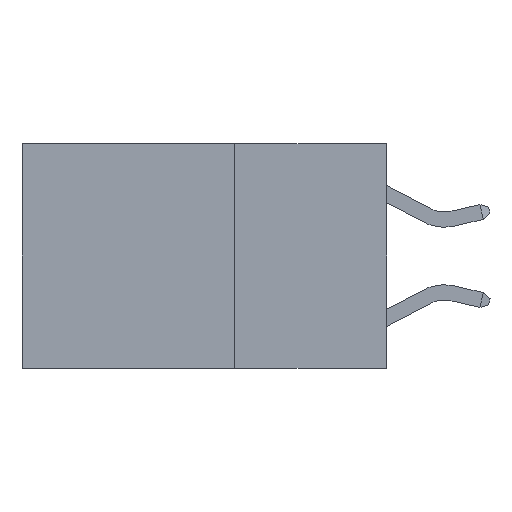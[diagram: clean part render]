
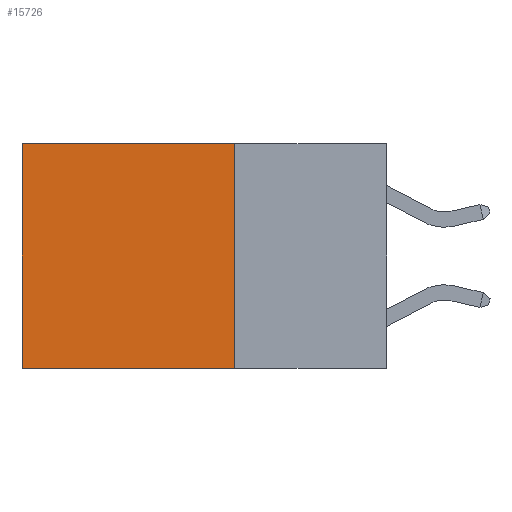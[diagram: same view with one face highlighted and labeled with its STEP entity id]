
A CAD part, left-side view. The second image highlights one B-rep face of the part: STEP entity #15726.
In plain terms, the highlighted planar face has unit normal (-1, 0, 0).
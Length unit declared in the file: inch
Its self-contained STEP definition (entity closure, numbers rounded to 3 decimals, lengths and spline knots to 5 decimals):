
#18 = DIRECTION ( 'NONE',  ( 0., 1., 0. ) ) ;
#278 = AXIS2_PLACEMENT_3D ( 'NONE', #5796, #12314, #14720 ) ;
#435 = CARTESIAN_POINT ( 'NONE',  ( 0.2625, 0.25, -0.37 ) ) ;
#825 = CARTESIAN_POINT ( 'NONE',  ( 0.2625, 0.6, 0. ) ) ;
#2890 = EDGE_CURVE ( 'NONE', #19317, #10851, #18489, .T. ) ;
#3599 = EDGE_LOOP ( 'NONE', ( #5713, #4068, #4902, #7153 ) ) ;
#4068 = ORIENTED_EDGE ( 'NONE', *, *, #8399, .F. ) ;
#4902 = ORIENTED_EDGE ( 'NONE', *, *, #13349, .F. ) ;
#5343 = VECTOR ( 'NONE', #9187, 39.37008 ) ;
#5713 = ORIENTED_EDGE ( 'NONE', *, *, #14063, .T. ) ;
#5796 = CARTESIAN_POINT ( 'NONE',  ( 0.2625, 0.25, 0. ) ) ;
#6402 = CARTESIAN_POINT ( 'NONE',  ( 0.2625, 0.25, 0. ) ) ;
#7153 = ORIENTED_EDGE ( 'NONE', *, *, #2890, .T. ) ;
#7994 = VERTEX_POINT ( 'NONE', #11801 ) ;
#8399 = EDGE_CURVE ( 'NONE', #13211, #7994, #14859, .T. ) ;
#9078 = LINE ( 'NONE', #825, #5343 ) ;
#9187 = DIRECTION ( 'NONE',  ( 0., 0., -1. ) ) ;
#10851 = VERTEX_POINT ( 'NONE', #14074 ) ;
#11346 = CARTESIAN_POINT ( 'NONE',  ( 0.2625, 0.25, 0. ) ) ;
#11454 = LINE ( 'NONE', #11346, #20994 ) ;
#11801 = CARTESIAN_POINT ( 'NONE',  ( 0.2625, 0.6, -0.37 ) ) ;
#12314 = DIRECTION ( 'NONE',  ( 1., 0., 0. ) ) ;
#13165 = DIRECTION ( 'NONE',  ( 0., 0., -1. ) ) ;
#13211 = VERTEX_POINT ( 'NONE', #20308 ) ;
#13349 = EDGE_CURVE ( 'NONE', #19317, #13211, #11454, .T. ) ;
#13593 = DIRECTION ( 'NONE',  ( 0., 1., 0. ) ) ;
#13909 = PLANE ( 'NONE',  #278 ) ;
#14032 = VECTOR ( 'NONE', #13593, 39.37008 ) ;
#14063 = EDGE_CURVE ( 'NONE', #10851, #7994, #9078, .T. ) ;
#14074 = CARTESIAN_POINT ( 'NONE',  ( 0.2625, 0.6, 0. ) ) ;
#14720 = DIRECTION ( 'NONE',  ( 0., 0., -1. ) ) ;
#14859 = LINE ( 'NONE', #435, #15783 ) ;
#15188 = CARTESIAN_POINT ( 'NONE',  ( 0.2625, 0.25, 0. ) ) ;
#15500 = FACE_OUTER_BOUND ( 'NONE', #3599, .T. ) ;
#15726 = ADVANCED_FACE ( 'NONE', ( #15500 ), #13909, .F. ) ;
#15783 = VECTOR ( 'NONE', #18, 39.37008 ) ;
#18489 = LINE ( 'NONE', #15188, #14032 ) ;
#19317 = VERTEX_POINT ( 'NONE', #6402 ) ;
#20308 = CARTESIAN_POINT ( 'NONE',  ( 0.2625, 0.25, -0.37 ) ) ;
#20994 = VECTOR ( 'NONE', #13165, 39.37008 ) ;
